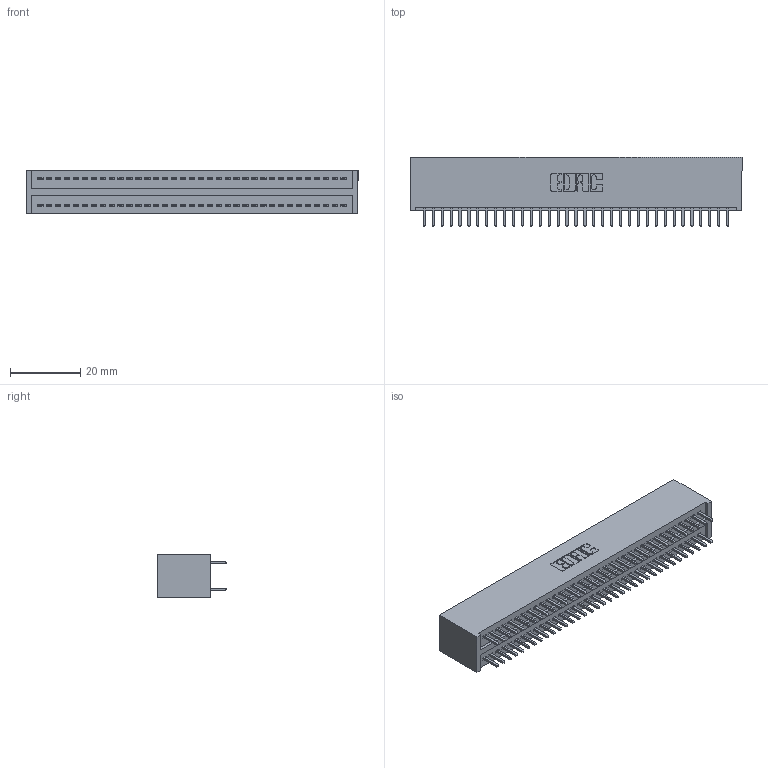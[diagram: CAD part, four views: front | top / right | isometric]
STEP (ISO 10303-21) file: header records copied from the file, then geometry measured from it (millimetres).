
FILE_DESCRIPTION (( 'STEP AP203' ), '1' );
FILE_NAME ('325-070-520-201.STEP', '2020-02-25T03:41:36', ( '' ), ( '' ), 'SwSTEP 2.0', 'SolidWorks 2016', '' );
FILE_SCHEMA (( 'CONFIG_CONTROL_DESIGN' ));
Length unit declared in the file: inch
Products named in the file (3): 325 Part_Lugless; 325-070-520-201; 325-292-001_325-293-120
Assembly tree (71 placements, depth 2):
  325-070-520-201
    325 Part_Lugless
    325-292-001_325-293-120  x70
Bounding box: 94.54 x 19.68 x 12.45 mm (x, y, z)
Volume: 12737.4 mm3; surface area: 15770.5 mm2
Topology: 71 solids, 71 shells, 3746 faces, 11137 edges, 7330 vertices
Faces by surface type: plane 2586, cylinder 1160
Entity records: 23163 total; most frequent: CARTESIAN_POINT 3846, ORIENTED_EDGE 3782, DIRECTION 3291, EDGE_CURVE 1891, LINE 1771, VECTOR 1771, VERTEX_POINT 1258, AXIS2_PLACEMENT_3D 760
